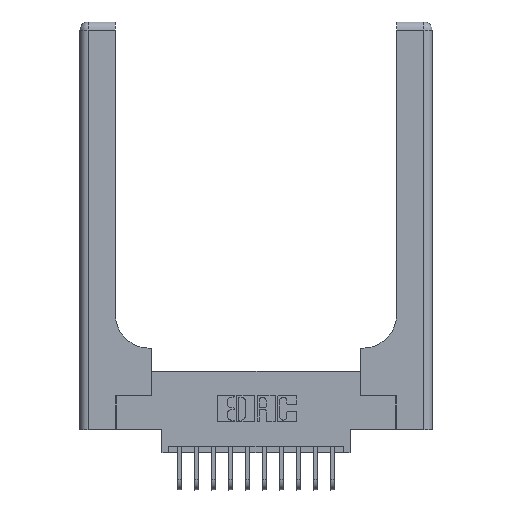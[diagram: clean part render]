
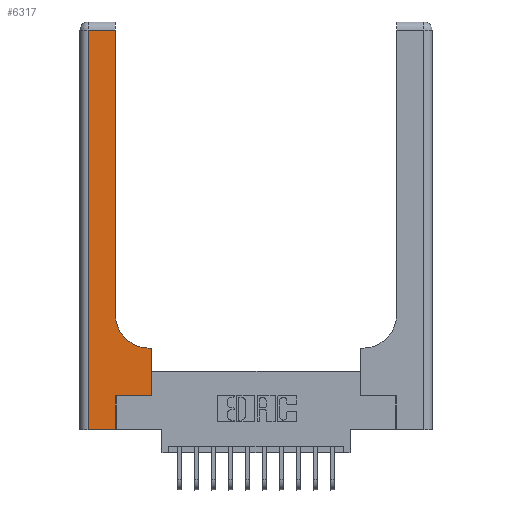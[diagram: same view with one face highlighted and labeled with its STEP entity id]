
A CAD part, top view. The second image highlights one B-rep face of the part: STEP entity #6317.
In plain terms, the highlighted planar face has unit normal (0, 0, 1).
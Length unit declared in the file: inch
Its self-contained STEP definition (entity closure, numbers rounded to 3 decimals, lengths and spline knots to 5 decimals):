
#44 = LINE ( 'NONE', #11402, #18302 ) ;
#414 = VECTOR ( 'NONE', #13346, 39.37008 ) ;
#502 = CARTESIAN_POINT ( 'NONE',  ( 0., 2.94, 0.37 ) ) ;
#657 = FACE_OUTER_BOUND ( 'NONE', #15123, .T. ) ;
#681 = DIRECTION ( 'NONE',  ( 0., 1., 0. ) ) ;
#685 = LINE ( 'NONE', #502, #5842 ) ;
#1216 = DIRECTION ( 'NONE',  ( -1., 0., 0. ) ) ;
#1442 = EDGE_CURVE ( 'NONE', #7160, #12246, #44, .T. ) ;
#1884 = ORIENTED_EDGE ( 'NONE', *, *, #8367, .T. ) ;
#1913 = EDGE_CURVE ( 'NONE', #12246, #14741, #3644, .T. ) ;
#2172 = CARTESIAN_POINT ( 'NONE',  ( 0.528, 0.25, 0.37 ) ) ;
#2263 = VECTOR ( 'NONE', #6845, 39.37008 ) ;
#2354 = DIRECTION ( 'NONE',  ( 1., 0., 0. ) ) ;
#2515 = LINE ( 'NONE', #12668, #11808 ) ;
#2880 = LINE ( 'NONE', #5399, #5649 ) ;
#2992 = DIRECTION ( 'NONE',  ( 1., 0., 0. ) ) ;
#3644 = LINE ( 'NONE', #16203, #414 ) ;
#3660 = LINE ( 'NONE', #2172, #8755 ) ;
#4309 = LINE ( 'NONE', #6928, #2263 ) ;
#4432 = CARTESIAN_POINT ( 'NONE',  ( 0.265, 0., 0.37 ) ) ;
#4507 = DIRECTION ( 'NONE',  ( 1., 0., 0. ) ) ;
#4543 = ORIENTED_EDGE ( 'NONE', *, *, #13901, .T. ) ;
#4848 = CARTESIAN_POINT ( 'NONE',  ( 0., 3., 0.37 ) ) ;
#5399 = CARTESIAN_POINT ( 'NONE',  ( 0.26, 0.6, 0.37 ) ) ;
#5649 = VECTOR ( 'NONE', #1216, 39.37008 ) ;
#5786 = CARTESIAN_POINT ( 'NONE',  ( 0.265, 0.25, 0.37 ) ) ;
#5842 = VECTOR ( 'NONE', #10831, 39.37008 ) ;
#5945 = CARTESIAN_POINT ( 'NONE',  ( 0.51, 0.6, 0.37 ) ) ;
#6317 = ADVANCED_FACE ( 'NONE', ( #657 ), #10624, .F. ) ;
#6480 = AXIS2_PLACEMENT_3D ( 'NONE', #9430, #14083, #2354 ) ;
#6623 = VERTEX_POINT ( 'NONE', #17639 ) ;
#6845 = DIRECTION ( 'NONE',  ( 0., 1., 0. ) ) ;
#6928 = CARTESIAN_POINT ( 'NONE',  ( 0.26, 3., 0.37 ) ) ;
#7160 = VERTEX_POINT ( 'NONE', #11086 ) ;
#7517 = VERTEX_POINT ( 'NONE', #17859 ) ;
#7867 = CARTESIAN_POINT ( 'NONE',  ( 0.26, 0.85, 0.37 ) ) ;
#7926 = DIRECTION ( 'NONE',  ( 0., 0., -1. ) ) ;
#8367 = EDGE_CURVE ( 'NONE', #6623, #15002, #685, .T. ) ;
#8590 = EDGE_CURVE ( 'NONE', #14741, #10338, #17234, .T. ) ;
#8755 = VECTOR ( 'NONE', #681, 39.37008 ) ;
#8818 = ORIENTED_EDGE ( 'NONE', *, *, #18206, .T. ) ;
#8836 = EDGE_CURVE ( 'NONE', #15002, #7160, #2515, .T. ) ;
#8863 = ORIENTED_EDGE ( 'NONE', *, *, #16446, .T. ) ;
#9211 = ORIENTED_EDGE ( 'NONE', *, *, #12888, .T. ) ;
#9430 = CARTESIAN_POINT ( 'NONE',  ( 0.51, 0.85, 0.37 ) ) ;
#9929 = ORIENTED_EDGE ( 'NONE', *, *, #1442, .T. ) ;
#10338 = VERTEX_POINT ( 'NONE', #16191 ) ;
#10624 = PLANE ( 'NONE',  #12033 ) ;
#10831 = DIRECTION ( 'NONE',  ( -1., 0., 0. ) ) ;
#11086 = CARTESIAN_POINT ( 'NONE',  ( 0.06, 0., 0.37 ) ) ;
#11402 = CARTESIAN_POINT ( 'NONE',  ( 0., 0., 0.37 ) ) ;
#11808 = VECTOR ( 'NONE', #15178, 39.37008 ) ;
#11836 = VERTEX_POINT ( 'NONE', #5945 ) ;
#12033 = AXIS2_PLACEMENT_3D ( 'NONE', #4848, #7926, #14813 ) ;
#12130 = CIRCLE ( 'NONE', #6480, 0.25 ) ;
#12246 = VERTEX_POINT ( 'NONE', #4432 ) ;
#12378 = ORIENTED_EDGE ( 'NONE', *, *, #8836, .T. ) ;
#12456 = ORIENTED_EDGE ( 'NONE', *, *, #8590, .T. ) ;
#12668 = CARTESIAN_POINT ( 'NONE',  ( 0.06, 3., 0.37 ) ) ;
#12888 = EDGE_CURVE ( 'NONE', #10338, #7517, #3660, .T. ) ;
#13346 = DIRECTION ( 'NONE',  ( 0., 1., 0. ) ) ;
#13901 = EDGE_CURVE ( 'NONE', #14831, #6623, #4309, .T. ) ;
#14083 = DIRECTION ( 'NONE',  ( 0., 0., -1. ) ) ;
#14741 = VERTEX_POINT ( 'NONE', #15951 ) ;
#14813 = DIRECTION ( 'NONE',  ( -1., 0., 0. ) ) ;
#14831 = VERTEX_POINT ( 'NONE', #7867 ) ;
#15002 = VERTEX_POINT ( 'NONE', #17989 ) ;
#15123 = EDGE_LOOP ( 'NONE', ( #4543, #1884, #12378, #9929, #17933, #12456, #9211, #8818, #8863 ) ) ;
#15178 = DIRECTION ( 'NONE',  ( 0., -1., 0. ) ) ;
#15951 = CARTESIAN_POINT ( 'NONE',  ( 0.265, 0.25, 0.37 ) ) ;
#16191 = CARTESIAN_POINT ( 'NONE',  ( 0.528, 0.25, 0.37 ) ) ;
#16203 = CARTESIAN_POINT ( 'NONE',  ( 0.265, 0., 0.37 ) ) ;
#16446 = EDGE_CURVE ( 'NONE', #11836, #14831, #12130, .T. ) ;
#17234 = LINE ( 'NONE', #5786, #18033 ) ;
#17639 = CARTESIAN_POINT ( 'NONE',  ( 0.26, 2.94, 0.37 ) ) ;
#17859 = CARTESIAN_POINT ( 'NONE',  ( 0.528, 0.6, 0.37 ) ) ;
#17933 = ORIENTED_EDGE ( 'NONE', *, *, #1913, .T. ) ;
#17989 = CARTESIAN_POINT ( 'NONE',  ( 0.06, 2.94, 0.37 ) ) ;
#18033 = VECTOR ( 'NONE', #2992, 39.37008 ) ;
#18206 = EDGE_CURVE ( 'NONE', #7517, #11836, #2880, .T. ) ;
#18302 = VECTOR ( 'NONE', #4507, 39.37008 ) ;
